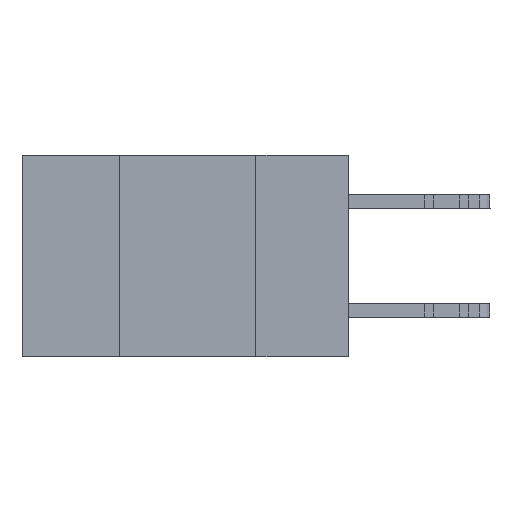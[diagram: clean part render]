
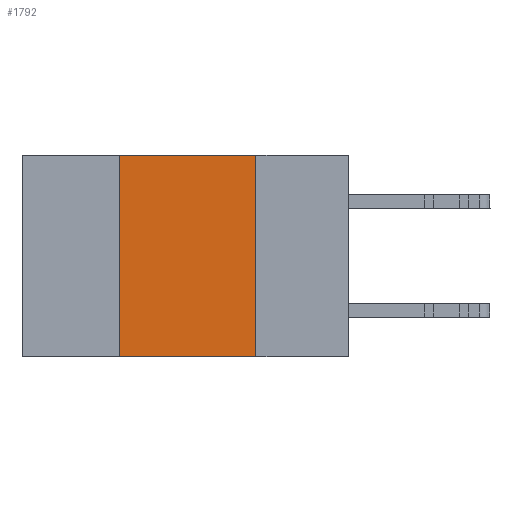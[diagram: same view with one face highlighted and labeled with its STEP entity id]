
A CAD part, left-side view. The second image highlights one B-rep face of the part: STEP entity #1792.
In plain terms, the highlighted planar face has unit normal (-1, 0, 0).
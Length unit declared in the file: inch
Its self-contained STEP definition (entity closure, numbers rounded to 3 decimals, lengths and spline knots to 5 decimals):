
#5 = VERTEX_POINT ( 'NONE', #24235 ) ;
#1114 = VERTEX_POINT ( 'NONE', #25543 ) ;
#1723 = VECTOR ( 'NONE', #20332, 39.37008 ) ;
#1792 = ADVANCED_FACE ( 'NONE', ( #26167 ), #23933, .F. ) ;
#2026 = EDGE_LOOP ( 'NONE', ( #20116, #24198, #12765, #6606 ) ) ;
#5762 = CARTESIAN_POINT ( 'NONE',  ( 0., 0.42, -0.37 ) ) ;
#6606 = ORIENTED_EDGE ( 'NONE', *, *, #7486, .T. ) ;
#7364 = LINE ( 'NONE', #16235, #1723 ) ;
#7486 = EDGE_CURVE ( 'NONE', #13907, #21311, #23726, .T. ) ;
#8867 = EDGE_CURVE ( 'NONE', #13907, #1114, #7364, .T. ) ;
#10230 = CARTESIAN_POINT ( 'NONE',  ( 0., 0.6, -0.37 ) ) ;
#10772 = VECTOR ( 'NONE', #19366, 39.37008 ) ;
#12750 = AXIS2_PLACEMENT_3D ( 'NONE', #18510, #15085, #15445 ) ;
#12765 = ORIENTED_EDGE ( 'NONE', *, *, #8867, .F. ) ;
#13907 = VERTEX_POINT ( 'NONE', #5762 ) ;
#14407 = EDGE_CURVE ( 'NONE', #1114, #5, #23417, .T. ) ;
#15085 = DIRECTION ( 'NONE',  ( 1., 0., 0. ) ) ;
#15445 = DIRECTION ( 'NONE',  ( 0., 0., -1. ) ) ;
#16222 = LINE ( 'NONE', #17337, #10772 ) ;
#16235 = CARTESIAN_POINT ( 'NONE',  ( 0., 0.42, -0.37 ) ) ;
#17337 = CARTESIAN_POINT ( 'NONE',  ( 0., 0.17, -0.37 ) ) ;
#18037 = VECTOR ( 'NONE', #23657, 39.37008 ) ;
#18356 = VECTOR ( 'NONE', #26383, 39.37008 ) ;
#18510 = CARTESIAN_POINT ( 'NONE',  ( 0., 0.6, 0. ) ) ;
#19323 = EDGE_CURVE ( 'NONE', #5, #21311, #16222, .T. ) ;
#19366 = DIRECTION ( 'NONE',  ( 0., 0., -1. ) ) ;
#20116 = ORIENTED_EDGE ( 'NONE', *, *, #19323, .F. ) ;
#20332 = DIRECTION ( 'NONE',  ( 0., 0., 1. ) ) ;
#21250 = CARTESIAN_POINT ( 'NONE',  ( 0., 0.17, -0.37 ) ) ;
#21311 = VERTEX_POINT ( 'NONE', #21250 ) ;
#21638 = CARTESIAN_POINT ( 'NONE',  ( 0., 0.6, 0. ) ) ;
#23417 = LINE ( 'NONE', #21638, #18037 ) ;
#23657 = DIRECTION ( 'NONE',  ( 0., -1., 0. ) ) ;
#23726 = LINE ( 'NONE', #10230, #18356 ) ;
#23933 = PLANE ( 'NONE',  #12750 ) ;
#24198 = ORIENTED_EDGE ( 'NONE', *, *, #14407, .F. ) ;
#24235 = CARTESIAN_POINT ( 'NONE',  ( 0., 0.17, 0. ) ) ;
#25543 = CARTESIAN_POINT ( 'NONE',  ( 0., 0.42, 0. ) ) ;
#26167 = FACE_OUTER_BOUND ( 'NONE', #2026, .T. ) ;
#26383 = DIRECTION ( 'NONE',  ( 0., -1., 0. ) ) ;
